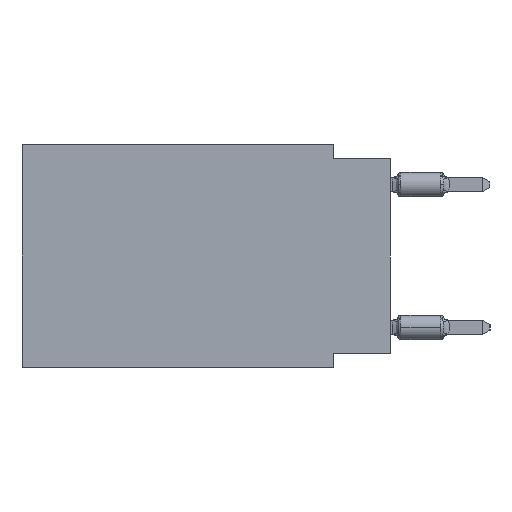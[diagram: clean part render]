
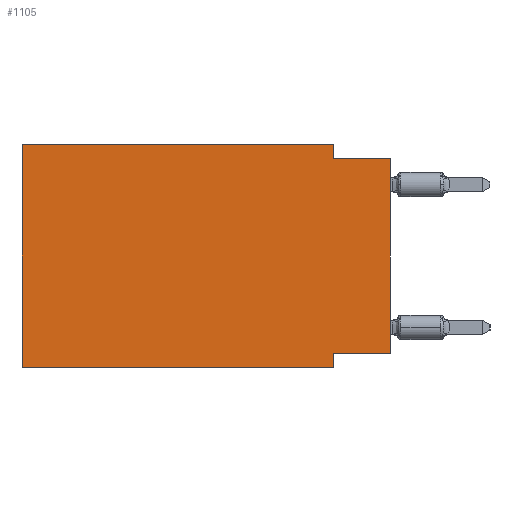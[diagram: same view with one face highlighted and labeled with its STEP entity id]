
A CAD part, left-side view. The second image highlights one B-rep face of the part: STEP entity #1105.
In plain terms, the highlighted planar face has unit normal (-1, 0, 0).
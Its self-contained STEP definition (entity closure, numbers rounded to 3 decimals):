
#137 = ORIENTED_EDGE ( 'NONE', *, *, #3676, .F. ) ;
#1018 = DIRECTION ( 'NONE',  ( 1., 0., 0. ) ) ;
#1105 = ADVANCED_FACE ( 'NONE', ( #23625 ), #3398, .F. ) ;
#1574 = CARTESIAN_POINT ( 'NONE',  ( 0., 0., 0. ) ) ;
#1959 = VERTEX_POINT ( 'NONE', #16725 ) ;
#2340 = LINE ( 'NONE', #20742, #16254 ) ;
#2580 = DIRECTION ( 'NONE',  ( 0., 0., 1. ) ) ;
#2759 = EDGE_CURVE ( 'NONE', #20858, #1959, #16612, .T. ) ;
#2820 = VECTOR ( 'NONE', #28870, 1000. ) ;
#3398 = PLANE ( 'NONE',  #6949 ) ;
#3676 = EDGE_CURVE ( 'NONE', #19683, #9397, #27550, .T. ) ;
#3902 = VERTEX_POINT ( 'NONE', #6708 ) ;
#4116 = VECTOR ( 'NONE', #14143, 1000. ) ;
#4932 = CARTESIAN_POINT ( 'NONE',  ( 0., 16.383, -9.906 ) ) ;
#5069 = CARTESIAN_POINT ( 'NONE',  ( 0., 0., -9.271 ) ) ;
#5153 = ORIENTED_EDGE ( 'NONE', *, *, #7970, .F. ) ;
#5388 = CARTESIAN_POINT ( 'NONE',  ( 0., 2.54, 0. ) ) ;
#5500 = EDGE_CURVE ( 'NONE', #19683, #24825, #24341, .T. ) ;
#6651 = ORIENTED_EDGE ( 'NONE', *, *, #17937, .T. ) ;
#6708 = CARTESIAN_POINT ( 'NONE',  ( 0., 2.54, -9.906 ) ) ;
#6949 = AXIS2_PLACEMENT_3D ( 'NONE', #7641, #1018, #26177 ) ;
#7212 = LINE ( 'NONE', #4932, #4116 ) ;
#7498 = VECTOR ( 'NONE', #8897, 1000. ) ;
#7641 = CARTESIAN_POINT ( 'NONE',  ( 0., 16.383, 0. ) ) ;
#7777 = CARTESIAN_POINT ( 'NONE',  ( 0., 2.54, 0. ) ) ;
#7970 = EDGE_CURVE ( 'NONE', #1959, #17160, #11670, .T. ) ;
#8897 = DIRECTION ( 'NONE',  ( 0., 0., -1. ) ) ;
#9397 = VERTEX_POINT ( 'NONE', #26591 ) ;
#10944 = ORIENTED_EDGE ( 'NONE', *, *, #28650, .F. ) ;
#11670 = LINE ( 'NONE', #21174, #19207 ) ;
#12630 = EDGE_LOOP ( 'NONE', ( #20582, #15600, #13502, #5153, #25546, #6651, #10944, #137 ) ) ;
#13502 = ORIENTED_EDGE ( 'NONE', *, *, #17876, .F. ) ;
#13961 = CARTESIAN_POINT ( 'NONE',  ( 0., 2.54, -0.635 ) ) ;
#14143 = DIRECTION ( 'NONE',  ( 0., -1., 0. ) ) ;
#14352 = CARTESIAN_POINT ( 'NONE',  ( 0., 16.383, 0. ) ) ;
#14590 = VERTEX_POINT ( 'NONE', #13961 ) ;
#14679 = CARTESIAN_POINT ( 'NONE',  ( 0., 0., -0.635 ) ) ;
#15600 = ORIENTED_EDGE ( 'NONE', *, *, #27194, .F. ) ;
#16254 = VECTOR ( 'NONE', #25552, 1000. ) ;
#16612 = LINE ( 'NONE', #14352, #21488 ) ;
#16711 = LINE ( 'NONE', #5388, #7498 ) ;
#16725 = CARTESIAN_POINT ( 'NONE',  ( 0., 16.383, 0. ) ) ;
#17160 = VERTEX_POINT ( 'NONE', #7777 ) ;
#17876 = EDGE_CURVE ( 'NONE', #17160, #14590, #16711, .T. ) ;
#17937 = EDGE_CURVE ( 'NONE', #20858, #3902, #7212, .T. ) ;
#19207 = VECTOR ( 'NONE', #21023, 1000. ) ;
#19642 = LINE ( 'NONE', #22871, #29173 ) ;
#19683 = VERTEX_POINT ( 'NONE', #21376 ) ;
#19855 = CARTESIAN_POINT ( 'NONE',  ( 0., 16.383, -9.906 ) ) ;
#20087 = VECTOR ( 'NONE', #20768, 1000. ) ;
#20316 = DIRECTION ( 'NONE',  ( 0., -1., 0. ) ) ;
#20582 = ORIENTED_EDGE ( 'NONE', *, *, #5500, .T. ) ;
#20742 = CARTESIAN_POINT ( 'NONE',  ( 0., 2.54, -9.906 ) ) ;
#20768 = DIRECTION ( 'NONE',  ( 0., 1., 0. ) ) ;
#20858 = VERTEX_POINT ( 'NONE', #19855 ) ;
#21023 = DIRECTION ( 'NONE',  ( 0., -1., 0. ) ) ;
#21174 = CARTESIAN_POINT ( 'NONE',  ( 0., 16.383, 0. ) ) ;
#21376 = CARTESIAN_POINT ( 'NONE',  ( 0., 0., -9.271 ) ) ;
#21488 = VECTOR ( 'NONE', #2580, 1000. ) ;
#22871 = CARTESIAN_POINT ( 'NONE',  ( 0., 0., -0.635 ) ) ;
#23625 = FACE_OUTER_BOUND ( 'NONE', #12630, .T. ) ;
#24341 = LINE ( 'NONE', #1574, #2820 ) ;
#24825 = VERTEX_POINT ( 'NONE', #14679 ) ;
#25546 = ORIENTED_EDGE ( 'NONE', *, *, #2759, .F. ) ;
#25552 = DIRECTION ( 'NONE',  ( 0., 0., -1. ) ) ;
#26177 = DIRECTION ( 'NONE',  ( 0., 0., -1. ) ) ;
#26591 = CARTESIAN_POINT ( 'NONE',  ( 0., 2.54, -9.271 ) ) ;
#27194 = EDGE_CURVE ( 'NONE', #14590, #24825, #19642, .T. ) ;
#27550 = LINE ( 'NONE', #5069, #20087 ) ;
#28650 = EDGE_CURVE ( 'NONE', #9397, #3902, #2340, .T. ) ;
#28870 = DIRECTION ( 'NONE',  ( 0., 0., 1. ) ) ;
#29173 = VECTOR ( 'NONE', #20316, 1000. ) ;
